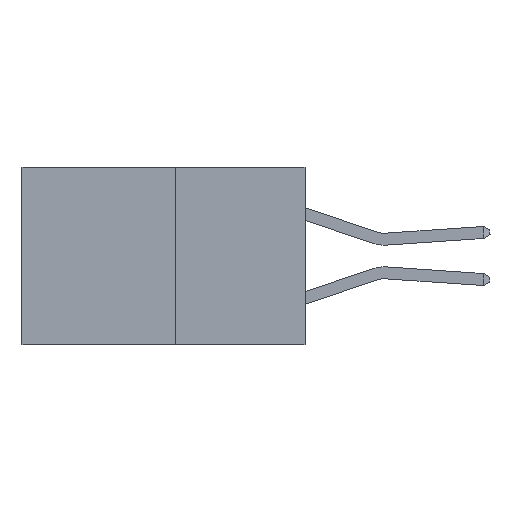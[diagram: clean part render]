
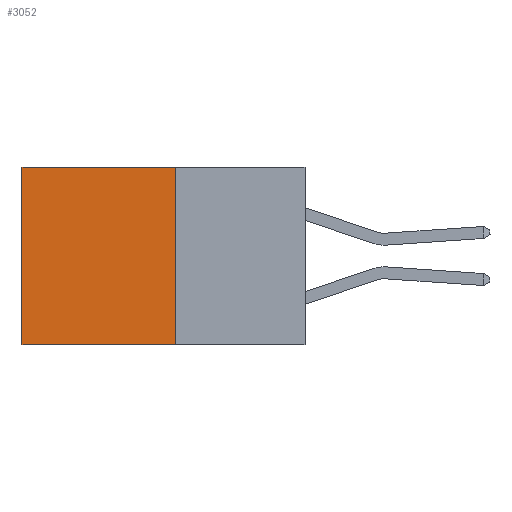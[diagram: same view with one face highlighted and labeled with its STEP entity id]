
A CAD part, left-side view. The second image highlights one B-rep face of the part: STEP entity #3052.
In plain terms, the highlighted planar face has unit normal (-1, 0, 0).
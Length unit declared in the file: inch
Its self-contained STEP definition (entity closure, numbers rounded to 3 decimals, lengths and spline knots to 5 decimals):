
#64 = EDGE_CURVE ( 'NONE', #676, #3054, #4477, .T. ) ;
#271 = VECTOR ( 'NONE', #6699, 39.37008 ) ;
#401 = CARTESIAN_POINT ( 'NONE',  ( 0.277, 0.59, 0. ) ) ;
#541 = CARTESIAN_POINT ( 'NONE',  ( 0.277, 0.27, -0.37 ) ) ;
#676 = VERTEX_POINT ( 'NONE', #9714 ) ;
#1404 = VECTOR ( 'NONE', #5552, 39.37008 ) ;
#2029 = EDGE_CURVE ( 'NONE', #676, #5135, #11734, .T. ) ;
#2665 = DIRECTION ( 'NONE',  ( 0., 0., -1. ) ) ;
#3052 = ADVANCED_FACE ( 'NONE', ( #5666 ), #10125, .F. ) ;
#3054 = VERTEX_POINT ( 'NONE', #401 ) ;
#4086 = ORIENTED_EDGE ( 'NONE', *, *, #2029, .F. ) ;
#4460 = CARTESIAN_POINT ( 'NONE',  ( 0.277, 0.27, 0. ) ) ;
#4477 = LINE ( 'NONE', #4460, #1404 ) ;
#5135 = VERTEX_POINT ( 'NONE', #10764 ) ;
#5534 = ORIENTED_EDGE ( 'NONE', *, *, #10649, .T. ) ;
#5552 = DIRECTION ( 'NONE',  ( 0., 1., 0. ) ) ;
#5666 = FACE_OUTER_BOUND ( 'NONE', #9377, .T. ) ;
#6165 = ORIENTED_EDGE ( 'NONE', *, *, #7936, .F. ) ;
#6664 = VECTOR ( 'NONE', #7760, 39.37008 ) ;
#6699 = DIRECTION ( 'NONE',  ( 0., 1., 0. ) ) ;
#7760 = DIRECTION ( 'NONE',  ( 0., 0., -1. ) ) ;
#7936 = EDGE_CURVE ( 'NONE', #5135, #12398, #13115, .T. ) ;
#8090 = AXIS2_PLACEMENT_3D ( 'NONE', #11199, #12192, #9244 ) ;
#8355 = LINE ( 'NONE', #9841, #13039 ) ;
#8505 = CARTESIAN_POINT ( 'NONE',  ( 0.277, 0.59, -0.37 ) ) ;
#8603 = CARTESIAN_POINT ( 'NONE',  ( 0.277, 0.27, -0.37 ) ) ;
#9244 = DIRECTION ( 'NONE',  ( 0., 0., -1. ) ) ;
#9377 = EDGE_LOOP ( 'NONE', ( #5534, #6165, #4086, #10175 ) ) ;
#9714 = CARTESIAN_POINT ( 'NONE',  ( 0.277, 0.27, 0. ) ) ;
#9841 = CARTESIAN_POINT ( 'NONE',  ( 0.277, 0.59, -0.37 ) ) ;
#10125 = PLANE ( 'NONE',  #8090 ) ;
#10175 = ORIENTED_EDGE ( 'NONE', *, *, #64, .T. ) ;
#10649 = EDGE_CURVE ( 'NONE', #3054, #12398, #8355, .T. ) ;
#10764 = CARTESIAN_POINT ( 'NONE',  ( 0.277, 0.27, -0.37 ) ) ;
#11199 = CARTESIAN_POINT ( 'NONE',  ( 0.277, 0.27, -0.37 ) ) ;
#11734 = LINE ( 'NONE', #8603, #6664 ) ;
#12192 = DIRECTION ( 'NONE',  ( 1., 0., 0. ) ) ;
#12398 = VERTEX_POINT ( 'NONE', #8505 ) ;
#13039 = VECTOR ( 'NONE', #2665, 39.37008 ) ;
#13115 = LINE ( 'NONE', #541, #271 ) ;
